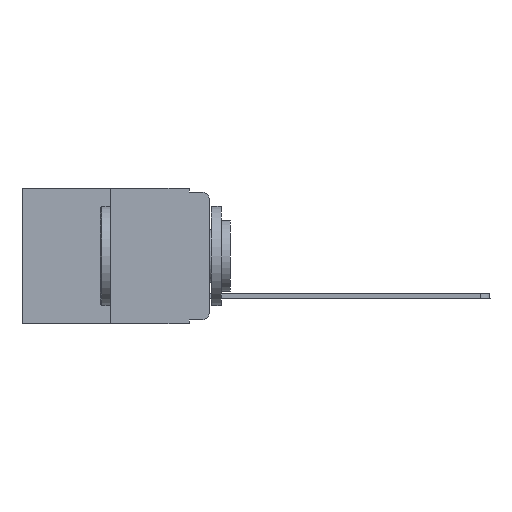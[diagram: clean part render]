
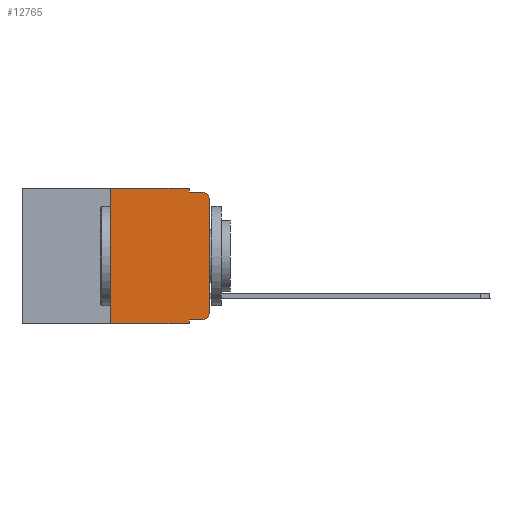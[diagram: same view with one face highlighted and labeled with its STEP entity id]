
A CAD part, left-side view. The second image highlights one B-rep face of the part: STEP entity #12765.
In plain terms, the highlighted planar face has unit normal (-1, 0, 0).
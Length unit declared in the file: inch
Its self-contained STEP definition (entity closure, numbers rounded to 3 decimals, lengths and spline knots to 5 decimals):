
#314 = VERTEX_POINT ( 'NONE', #11859 ) ;
#875 = VECTOR ( 'NONE', #3509, 39.37008 ) ;
#906 = VECTOR ( 'NONE', #16552, 39.37008 ) ;
#1552 = CIRCLE ( 'NONE', #10338, 0.02 ) ;
#1847 = CARTESIAN_POINT ( 'NONE',  ( 0., 0.051, -0.01 ) ) ;
#2628 = VECTOR ( 'NONE', #9617, 39.37008 ) ;
#2871 = VERTEX_POINT ( 'NONE', #11991 ) ;
#3166 = VECTOR ( 'NONE', #14834, 39.37008 ) ;
#3390 = CARTESIAN_POINT ( 'NONE',  ( 0., 0.051, -0.01 ) ) ;
#3509 = DIRECTION ( 'NONE',  ( 0., 0., -1. ) ) ;
#3652 = PLANE ( 'NONE',  #10693 ) ;
#3687 = CARTESIAN_POINT ( 'NONE',  ( 0., 0., -0.313 ) ) ;
#3816 = CARTESIAN_POINT ( 'NONE',  ( 0., 0.02, -0.333 ) ) ;
#4691 = LINE ( 'NONE', #18184, #875 ) ;
#4978 = CARTESIAN_POINT ( 'NONE',  ( 0., 0.25, 0. ) ) ;
#4997 = VECTOR ( 'NONE', #17671, 39.37008 ) ;
#5465 = DIRECTION ( 'NONE',  ( 0., -1., 0. ) ) ;
#5474 = EDGE_CURVE ( 'NONE', #9756, #17501, #6551, .T. ) ;
#5752 = VERTEX_POINT ( 'NONE', #9517 ) ;
#6090 = ORIENTED_EDGE ( 'NONE', *, *, #7210, .T. ) ;
#6170 = EDGE_CURVE ( 'NONE', #17501, #11153, #1552, .T. ) ;
#6291 = EDGE_CURVE ( 'NONE', #8448, #9756, #14178, .T. ) ;
#6431 = EDGE_CURVE ( 'NONE', #14909, #314, #10343, .T. ) ;
#6551 = LINE ( 'NONE', #14771, #3166 ) ;
#7106 = ORIENTED_EDGE ( 'NONE', *, *, #5474, .T. ) ;
#7210 = EDGE_CURVE ( 'NONE', #14909, #5752, #18580, .T. ) ;
#7882 = VERTEX_POINT ( 'NONE', #3390 ) ;
#8421 = CARTESIAN_POINT ( 'NONE',  ( 0., 0., -0.03 ) ) ;
#8448 = VERTEX_POINT ( 'NONE', #3816 ) ;
#8453 = ORIENTED_EDGE ( 'NONE', *, *, #11832, .F. ) ;
#8558 = ORIENTED_EDGE ( 'NONE', *, *, #6170, .T. ) ;
#8571 = EDGE_CURVE ( 'NONE', #314, #2871, #16952, .T. ) ;
#8586 = ORIENTED_EDGE ( 'NONE', *, *, #6291, .T. ) ;
#8662 = DIRECTION ( 'NONE',  ( 0., 0., -1. ) ) ;
#8778 = LINE ( 'NONE', #17797, #4997 ) ;
#8850 = CARTESIAN_POINT ( 'NONE',  ( 0., 0.25, -0.343 ) ) ;
#9449 = DIRECTION ( 'NONE',  ( 0., 0., -1. ) ) ;
#9517 = CARTESIAN_POINT ( 'NONE',  ( 0., 0.051, -0.343 ) ) ;
#9549 = LINE ( 'NONE', #1847, #11822 ) ;
#9617 = DIRECTION ( 'NONE',  ( 0., 0., -1. ) ) ;
#9747 = CARTESIAN_POINT ( 'NONE',  ( 0., 0.051, -0.333 ) ) ;
#9756 = VERTEX_POINT ( 'NONE', #3687 ) ;
#9815 = CARTESIAN_POINT ( 'NONE',  ( 0., 0.02, -0.01 ) ) ;
#10120 = ORIENTED_EDGE ( 'NONE', *, *, #15307, .F. ) ;
#10338 = AXIS2_PLACEMENT_3D ( 'NONE', #17365, #12979, #8662 ) ;
#10343 = LINE ( 'NONE', #4978, #906 ) ;
#10567 = DIRECTION ( 'NONE',  ( 0., 0., -1. ) ) ;
#10693 = AXIS2_PLACEMENT_3D ( 'NONE', #18341, #12360, #9449 ) ;
#10866 = VECTOR ( 'NONE', #5465, 39.37008 ) ;
#11153 = VERTEX_POINT ( 'NONE', #9815 ) ;
#11822 = VECTOR ( 'NONE', #14928, 39.37008 ) ;
#11832 = EDGE_CURVE ( 'NONE', #2871, #7882, #14093, .T. ) ;
#11859 = CARTESIAN_POINT ( 'NONE',  ( 0., 0.25, 0. ) ) ;
#11991 = CARTESIAN_POINT ( 'NONE',  ( 0., 0.051, 0. ) ) ;
#12360 = DIRECTION ( 'NONE',  ( 1., 0., 0. ) ) ;
#12765 = ADVANCED_FACE ( 'NONE', ( #16933 ), #3652, .F. ) ;
#12979 = DIRECTION ( 'NONE',  ( -1., 0., 0. ) ) ;
#13289 = DIRECTION ( 'NONE',  ( -1., 0., 0. ) ) ;
#13426 = EDGE_CURVE ( 'NONE', #17340, #5752, #4691, .T. ) ;
#13744 = CARTESIAN_POINT ( 'NONE',  ( 0., 0.051, 0. ) ) ;
#14093 = LINE ( 'NONE', #13744, #2628 ) ;
#14095 = CARTESIAN_POINT ( 'NONE',  ( 0., 0.473, -0.343 ) ) ;
#14178 = CIRCLE ( 'NONE', #16192, 0.02 ) ;
#14206 = VECTOR ( 'NONE', #16942, 39.37008 ) ;
#14523 = ORIENTED_EDGE ( 'NONE', *, *, #13426, .F. ) ;
#14771 = CARTESIAN_POINT ( 'NONE',  ( 0., 0., 0. ) ) ;
#14834 = DIRECTION ( 'NONE',  ( 0., 0., 1. ) ) ;
#14909 = VERTEX_POINT ( 'NONE', #8850 ) ;
#14928 = DIRECTION ( 'NONE',  ( 0., -1., 0. ) ) ;
#15307 = EDGE_CURVE ( 'NONE', #7882, #11153, #9549, .T. ) ;
#15449 = CARTESIAN_POINT ( 'NONE',  ( 0., 0.473, 0. ) ) ;
#16192 = AXIS2_PLACEMENT_3D ( 'NONE', #17925, #13289, #10567 ) ;
#16230 = ORIENTED_EDGE ( 'NONE', *, *, #17123, .T. ) ;
#16552 = DIRECTION ( 'NONE',  ( 0., 0., 1. ) ) ;
#16933 = FACE_OUTER_BOUND ( 'NONE', #17964, .T. ) ;
#16942 = DIRECTION ( 'NONE',  ( 0., -1., 0. ) ) ;
#16952 = LINE ( 'NONE', #15449, #14206 ) ;
#17082 = ORIENTED_EDGE ( 'NONE', *, *, #8571, .F. ) ;
#17091 = ORIENTED_EDGE ( 'NONE', *, *, #6431, .F. ) ;
#17123 = EDGE_CURVE ( 'NONE', #17340, #8448, #8778, .T. ) ;
#17340 = VERTEX_POINT ( 'NONE', #9747 ) ;
#17365 = CARTESIAN_POINT ( 'NONE',  ( 0., 0.02, -0.03 ) ) ;
#17501 = VERTEX_POINT ( 'NONE', #8421 ) ;
#17671 = DIRECTION ( 'NONE',  ( 0., -1., 0. ) ) ;
#17797 = CARTESIAN_POINT ( 'NONE',  ( 0., 0.051, -0.333 ) ) ;
#17925 = CARTESIAN_POINT ( 'NONE',  ( 0., 0.02, -0.313 ) ) ;
#17964 = EDGE_LOOP ( 'NONE', ( #7106, #8558, #10120, #8453, #17082, #17091, #6090, #14523, #16230, #8586 ) ) ;
#18184 = CARTESIAN_POINT ( 'NONE',  ( 0., 0.051, 0. ) ) ;
#18341 = CARTESIAN_POINT ( 'NONE',  ( 0., 0.473, 0. ) ) ;
#18580 = LINE ( 'NONE', #14095, #10866 ) ;
